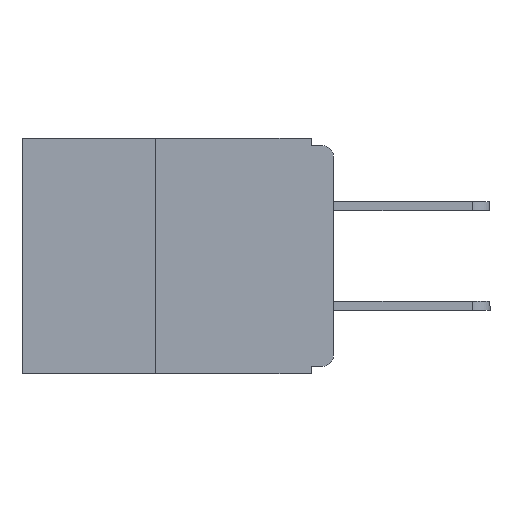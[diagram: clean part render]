
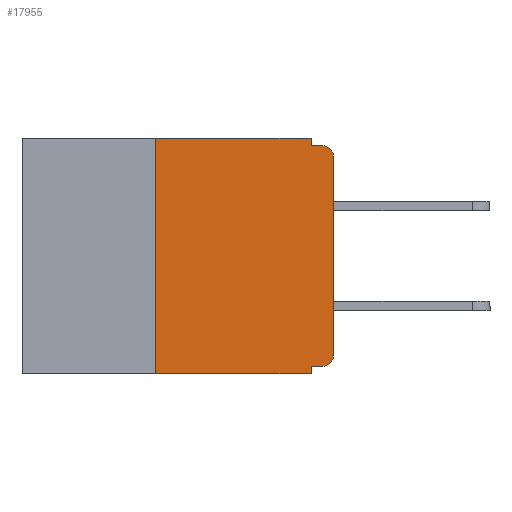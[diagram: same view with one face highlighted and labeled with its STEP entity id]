
A CAD part, left-side view. The second image highlights one B-rep face of the part: STEP entity #17955.
In plain terms, the highlighted planar face has unit normal (-1, 0, 0).
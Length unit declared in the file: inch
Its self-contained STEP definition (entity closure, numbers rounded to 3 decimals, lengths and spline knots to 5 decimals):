
#159 = VERTEX_POINT ( 'NONE', #4720 ) ;
#637 = VECTOR ( 'NONE', #8544, 39.37008 ) ;
#885 = EDGE_CURVE ( 'NONE', #14635, #159, #20248, .T. ) ;
#938 = DIRECTION ( 'NONE',  ( 0., 0., -1. ) ) ;
#1057 = AXIS2_PLACEMENT_3D ( 'NONE', #16317, #4240, #18383 ) ;
#1465 = EDGE_CURVE ( 'NONE', #20318, #12654, #12965, .T. ) ;
#2889 = EDGE_CURVE ( 'NONE', #12584, #6198, #16957, .T. ) ;
#3110 = VECTOR ( 'NONE', #7358, 39.37008 ) ;
#3712 = CARTESIAN_POINT ( 'NONE',  ( 0., 0.015, -0.01 ) ) ;
#4240 = DIRECTION ( 'NONE',  ( -1., 0., 0. ) ) ;
#4720 = CARTESIAN_POINT ( 'NONE',  ( 0., 0.031, -0.01 ) ) ;
#4828 = CARTESIAN_POINT ( 'NONE',  ( 0., 0.031, 0. ) ) ;
#5213 = CARTESIAN_POINT ( 'NONE',  ( 0., 0.015, -0.32 ) ) ;
#5536 = ORIENTED_EDGE ( 'NONE', *, *, #5698, .T. ) ;
#5590 = ORIENTED_EDGE ( 'NONE', *, *, #15087, .T. ) ;
#5663 = VERTEX_POINT ( 'NONE', #18621 ) ;
#5698 = EDGE_CURVE ( 'NONE', #9442, #5663, #25915, .T. ) ;
#6118 = CARTESIAN_POINT ( 'NONE',  ( 0., 0.25, -0.33 ) ) ;
#6198 = VERTEX_POINT ( 'NONE', #8013 ) ;
#6509 = ORIENTED_EDGE ( 'NONE', *, *, #11256, .F. ) ;
#6811 = CARTESIAN_POINT ( 'NONE',  ( 0., 0.031, -0.33 ) ) ;
#7358 = DIRECTION ( 'NONE',  ( 0., -1., 0. ) ) ;
#7573 = VECTOR ( 'NONE', #8645, 39.37008 ) ;
#7576 = EDGE_CURVE ( 'NONE', #6198, #14635, #18262, .T. ) ;
#7627 = VERTEX_POINT ( 'NONE', #6811 ) ;
#7669 = ORIENTED_EDGE ( 'NONE', *, *, #885, .F. ) ;
#8010 = DIRECTION ( 'NONE',  ( 0., 0., -1. ) ) ;
#8013 = CARTESIAN_POINT ( 'NONE',  ( 0., 0.25, 0. ) ) ;
#8544 = DIRECTION ( 'NONE',  ( 0., 0., 1. ) ) ;
#8645 = DIRECTION ( 'NONE',  ( 0., -1., 0. ) ) ;
#9189 = CARTESIAN_POINT ( 'NONE',  ( 0., 0., -0.305 ) ) ;
#9442 = VERTEX_POINT ( 'NONE', #9189 ) ;
#9549 = VECTOR ( 'NONE', #14320, 39.37008 ) ;
#10105 = DIRECTION ( 'NONE',  ( -1., 0., 0. ) ) ;
#10183 = VECTOR ( 'NONE', #17725, 39.37008 ) ;
#10318 = CARTESIAN_POINT ( 'NONE',  ( 0., 0.031, -0.32 ) ) ;
#10911 = CARTESIAN_POINT ( 'NONE',  ( 0., 0.25, -0.33 ) ) ;
#11256 = EDGE_CURVE ( 'NONE', #159, #24283, #24469, .T. ) ;
#11813 = ORIENTED_EDGE ( 'NONE', *, *, #7576, .F. ) ;
#11887 = ORIENTED_EDGE ( 'NONE', *, *, #2889, .F. ) ;
#11956 = PLANE ( 'NONE',  #17401 ) ;
#12584 = VERTEX_POINT ( 'NONE', #6118 ) ;
#12654 = VERTEX_POINT ( 'NONE', #10318 ) ;
#12965 = LINE ( 'NONE', #18246, #17686 ) ;
#13434 = ORIENTED_EDGE ( 'NONE', *, *, #14305, .T. ) ;
#13435 = CARTESIAN_POINT ( 'NONE',  ( 0., 0.031, 0. ) ) ;
#13980 = ORIENTED_EDGE ( 'NONE', *, *, #17724, .F. ) ;
#14305 = EDGE_CURVE ( 'NONE', #12584, #7627, #23437, .T. ) ;
#14320 = DIRECTION ( 'NONE',  ( 0., 0., -1. ) ) ;
#14635 = VERTEX_POINT ( 'NONE', #4828 ) ;
#14757 = EDGE_LOOP ( 'NONE', ( #5536, #5590, #6509, #7669, #11813, #11887, #13434, #13980, #14876, #19500 ) ) ;
#14876 = ORIENTED_EDGE ( 'NONE', *, *, #1465, .F. ) ;
#15087 = EDGE_CURVE ( 'NONE', #5663, #24283, #15324, .T. ) ;
#15324 = CIRCLE ( 'NONE', #1057, 0.015 ) ;
#15820 = CARTESIAN_POINT ( 'NONE',  ( 0., 0.437, -0.33 ) ) ;
#15955 = CARTESIAN_POINT ( 'NONE',  ( 0., 0.437, 0. ) ) ;
#16317 = CARTESIAN_POINT ( 'NONE',  ( 0., 0.015, -0.025 ) ) ;
#16957 = LINE ( 'NONE', #10911, #637 ) ;
#16998 = DIRECTION ( 'NONE',  ( 0., 1., 0. ) ) ;
#17352 = CARTESIAN_POINT ( 'NONE',  ( 0., 0., -0.01 ) ) ;
#17401 = AXIS2_PLACEMENT_3D ( 'NONE', #15955, #20044, #8010 ) ;
#17686 = VECTOR ( 'NONE', #16998, 39.37008 ) ;
#17724 = EDGE_CURVE ( 'NONE', #12654, #7627, #24372, .T. ) ;
#17725 = DIRECTION ( 'NONE',  ( 0., 0., 1. ) ) ;
#17802 = CARTESIAN_POINT ( 'NONE',  ( 0., 0., 0. ) ) ;
#17887 = DIRECTION ( 'NONE',  ( 0., -1., 0. ) ) ;
#17955 = ADVANCED_FACE ( 'NONE', ( #19525 ), #11956, .F. ) ;
#18218 = AXIS2_PLACEMENT_3D ( 'NONE', #22107, #10105, #23993 ) ;
#18246 = CARTESIAN_POINT ( 'NONE',  ( 0., 0., -0.32 ) ) ;
#18262 = LINE ( 'NONE', #18668, #7573 ) ;
#18383 = DIRECTION ( 'NONE',  ( 0., 0., -1. ) ) ;
#18621 = CARTESIAN_POINT ( 'NONE',  ( 0., 0., -0.025 ) ) ;
#18668 = CARTESIAN_POINT ( 'NONE',  ( 0., 0.437, 0. ) ) ;
#19340 = CARTESIAN_POINT ( 'NONE',  ( 0., 0.031, -0.33 ) ) ;
#19500 = ORIENTED_EDGE ( 'NONE', *, *, #25377, .T. ) ;
#19525 = FACE_OUTER_BOUND ( 'NONE', #14757, .T. ) ;
#19856 = VECTOR ( 'NONE', #938, 39.37008 ) ;
#20044 = DIRECTION ( 'NONE',  ( 1., 0., 0. ) ) ;
#20248 = LINE ( 'NONE', #13435, #9549 ) ;
#20318 = VERTEX_POINT ( 'NONE', #5213 ) ;
#20345 = CIRCLE ( 'NONE', #18218, 0.015 ) ;
#22107 = CARTESIAN_POINT ( 'NONE',  ( 0., 0.015, -0.305 ) ) ;
#22853 = VECTOR ( 'NONE', #17887, 39.37008 ) ;
#23437 = LINE ( 'NONE', #15820, #22853 ) ;
#23993 = DIRECTION ( 'NONE',  ( 0., 0., -1. ) ) ;
#24283 = VERTEX_POINT ( 'NONE', #3712 ) ;
#24372 = LINE ( 'NONE', #19340, #19856 ) ;
#24469 = LINE ( 'NONE', #17352, #3110 ) ;
#25377 = EDGE_CURVE ( 'NONE', #20318, #9442, #20345, .T. ) ;
#25915 = LINE ( 'NONE', #17802, #10183 ) ;
